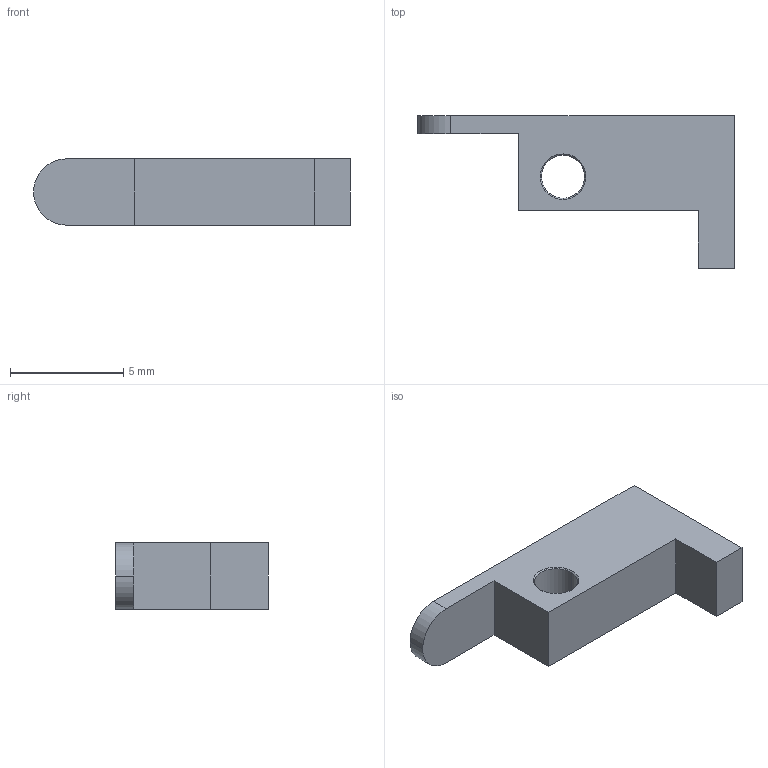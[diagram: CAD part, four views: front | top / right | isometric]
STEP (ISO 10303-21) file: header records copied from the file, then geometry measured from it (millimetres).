
FILE_DESCRIPTION (( 'STEP AP214' ), '1' );
FILE_NAME ('LOADED CHAMBER INDICATOR.STEP', '2013-06-19T14:01:45', ( 'Asher' ), ( '' ), 'SwSTEP 2.0', 'SolidWorks 2013', '' );
FILE_SCHEMA (( 'AUTOMOTIVE_DESIGN' ));
Length unit declared in the file: millimetre
Products named in the file (1): LOADED CHAMBER INDICATOR
Bounding box: 13.97 x 6.73 x 2.92 mm (x, y, z)
Volume: 129.6 mm3; surface area: 224.5 mm2
Topology: 1 solids, 1 shells, 17 faces, 41 edges, 26 vertices
Faces by surface type: plane 9, cone 4, cylinder 4
Entity records: 533 total; most frequent: DIRECTION 89, CARTESIAN_POINT 85, ORIENTED_EDGE 82, EDGE_CURVE 41, AXIS2_PLACEMENT_3D 30, LINE 29, VECTOR 29, VERTEX_POINT 26
